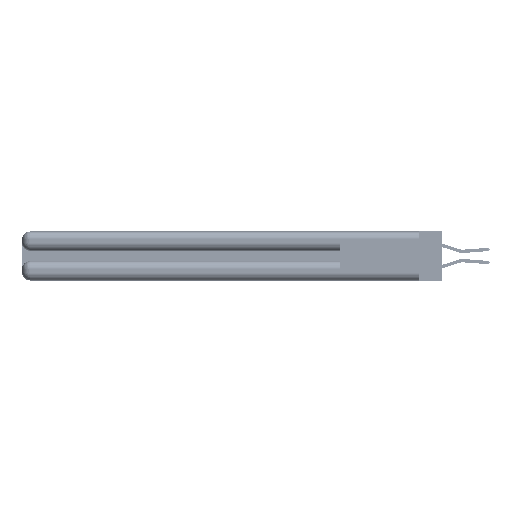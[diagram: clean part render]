
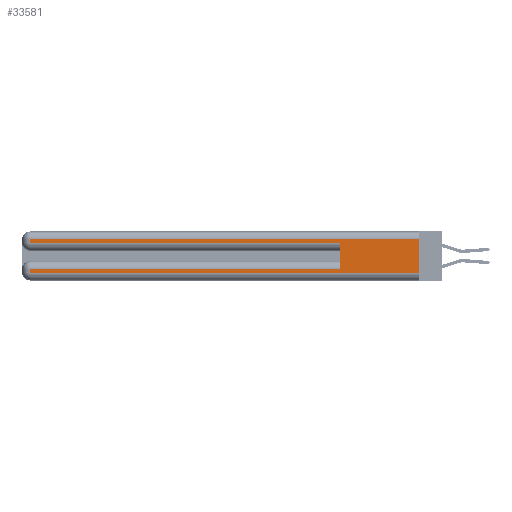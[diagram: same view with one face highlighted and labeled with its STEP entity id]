
A CAD part, left-side view. The second image highlights one B-rep face of the part: STEP entity #33581.
In plain terms, the highlighted planar face has unit normal (-1, 0, 0).
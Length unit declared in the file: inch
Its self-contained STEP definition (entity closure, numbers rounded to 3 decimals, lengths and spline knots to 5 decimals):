
#371 = AXIS2_PLACEMENT_3D ( 'NONE', #20050, #43088, #12619 ) ;
#1515 = EDGE_CURVE ( 'NONE', #23495, #11359, #19067, .T. ) ;
#2135 = LINE ( 'NONE', #46785, #49922 ) ;
#2310 = EDGE_CURVE ( 'NONE', #23495, #14237, #45038, .T. ) ;
#3521 = EDGE_LOOP ( 'NONE', ( #29704, #23297, #36366, #34885, #6867, #40385, #10785, #37688 ) ) ;
#4429 = VECTOR ( 'NONE', #42949, 39.37008 ) ;
#4599 = CARTESIAN_POINT ( 'NONE',  ( 0., 0.6, 0.085 ) ) ;
#6366 = EDGE_CURVE ( 'NONE', #27549, #14237, #40799, .T. ) ;
#6867 = ORIENTED_EDGE ( 'NONE', *, *, #22589, .F. ) ;
#8176 = CARTESIAN_POINT ( 'NONE',  ( 0., 0., 0.31 ) ) ;
#8866 = CARTESIAN_POINT ( 'NONE',  ( 0., 2.94, 0.31 ) ) ;
#9903 = VECTOR ( 'NONE', #34105, 39.37008 ) ;
#10785 = ORIENTED_EDGE ( 'NONE', *, *, #44476, .T. ) ;
#11359 = VERTEX_POINT ( 'NONE', #8866 ) ;
#11719 = VECTOR ( 'NONE', #46398, 39.37008 ) ;
#12106 = DIRECTION ( 'NONE',  ( 0., 1., 0. ) ) ;
#12396 = CARTESIAN_POINT ( 'NONE',  ( 0., 2.94, 0.37 ) ) ;
#12619 = DIRECTION ( 'NONE',  ( 0., 0., -1. ) ) ;
#14237 = VERTEX_POINT ( 'NONE', #34936 ) ;
#14288 = VERTEX_POINT ( 'NONE', #4599 ) ;
#14501 = CARTESIAN_POINT ( 'NONE',  ( 0., 0.6, 0.145 ) ) ;
#16341 = CARTESIAN_POINT ( 'NONE',  ( 0., 2.94, 0.37 ) ) ;
#16879 = EDGE_CURVE ( 'NONE', #11359, #45837, #44421, .T. ) ;
#17251 = DIRECTION ( 'NONE',  ( 0., 0., -1. ) ) ;
#19067 = LINE ( 'NONE', #27681, #48704 ) ;
#20050 = CARTESIAN_POINT ( 'NONE',  ( 0., 0., 0.37 ) ) ;
#21018 = CARTESIAN_POINT ( 'NONE',  ( 0., 0.6, 0.285 ) ) ;
#22589 = EDGE_CURVE ( 'NONE', #14288, #27505, #44075, .T. ) ;
#23297 = ORIENTED_EDGE ( 'NONE', *, *, #1515, .T. ) ;
#23495 = VERTEX_POINT ( 'NONE', #8176 ) ;
#24059 = DIRECTION ( 'NONE',  ( 0., 0., -1. ) ) ;
#27158 = CARTESIAN_POINT ( 'NONE',  ( 0., 2.94, 0.085 ) ) ;
#27397 = VERTEX_POINT ( 'NONE', #27158 ) ;
#27505 = VERTEX_POINT ( 'NONE', #21018 ) ;
#27549 = VERTEX_POINT ( 'NONE', #39990 ) ;
#27681 = CARTESIAN_POINT ( 'NONE',  ( 0., 0., 0.31 ) ) ;
#28729 = VECTOR ( 'NONE', #17251, 39.37008 ) ;
#29397 = FACE_OUTER_BOUND ( 'NONE', #3521, .T. ) ;
#29704 = ORIENTED_EDGE ( 'NONE', *, *, #2310, .F. ) ;
#29876 = VECTOR ( 'NONE', #24059, 39.37008 ) ;
#31416 = DIRECTION ( 'NONE',  ( 0., 1., 0. ) ) ;
#33535 = EDGE_CURVE ( 'NONE', #14288, #27397, #2135, .T. ) ;
#33581 = ADVANCED_FACE ( 'NONE', ( #29397 ), #43593, .F. ) ;
#34105 = DIRECTION ( 'NONE',  ( 0., -1., 0. ) ) ;
#34186 = EDGE_CURVE ( 'NONE', #45837, #27505, #40194, .T. ) ;
#34885 = ORIENTED_EDGE ( 'NONE', *, *, #34186, .T. ) ;
#34936 = CARTESIAN_POINT ( 'NONE',  ( 0., 0., 0.06 ) ) ;
#36239 = CARTESIAN_POINT ( 'NONE',  ( 0., 0., 0.37 ) ) ;
#36366 = ORIENTED_EDGE ( 'NONE', *, *, #16879, .T. ) ;
#37688 = ORIENTED_EDGE ( 'NONE', *, *, #6366, .T. ) ;
#37730 = DIRECTION ( 'NONE',  ( 0., 0., 1. ) ) ;
#39990 = CARTESIAN_POINT ( 'NONE',  ( 0., 2.94, 0.06 ) ) ;
#40092 = CARTESIAN_POINT ( 'NONE',  ( 0., 2.94, 0.285 ) ) ;
#40194 = LINE ( 'NONE', #42528, #11719 ) ;
#40385 = ORIENTED_EDGE ( 'NONE', *, *, #33535, .T. ) ;
#40799 = LINE ( 'NONE', #41372, #9903 ) ;
#41035 = VECTOR ( 'NONE', #37730, 39.37008 ) ;
#41372 = CARTESIAN_POINT ( 'NONE',  ( 0., 0., 0.06 ) ) ;
#41989 = LINE ( 'NONE', #16341, #4429 ) ;
#42528 = CARTESIAN_POINT ( 'NONE',  ( 0., 0., 0.285 ) ) ;
#42949 = DIRECTION ( 'NONE',  ( 0., 0., -1. ) ) ;
#43088 = DIRECTION ( 'NONE',  ( 1., 0., 0. ) ) ;
#43593 = PLANE ( 'NONE',  #371 ) ;
#44075 = LINE ( 'NONE', #14501, #41035 ) ;
#44421 = LINE ( 'NONE', #12396, #29876 ) ;
#44476 = EDGE_CURVE ( 'NONE', #27397, #27549, #41989, .T. ) ;
#45038 = LINE ( 'NONE', #36239, #28729 ) ;
#45837 = VERTEX_POINT ( 'NONE', #40092 ) ;
#46398 = DIRECTION ( 'NONE',  ( 0., -1., 0. ) ) ;
#46785 = CARTESIAN_POINT ( 'NONE',  ( 0., 0., 0.085 ) ) ;
#48704 = VECTOR ( 'NONE', #31416, 39.37008 ) ;
#49922 = VECTOR ( 'NONE', #12106, 39.37008 ) ;
